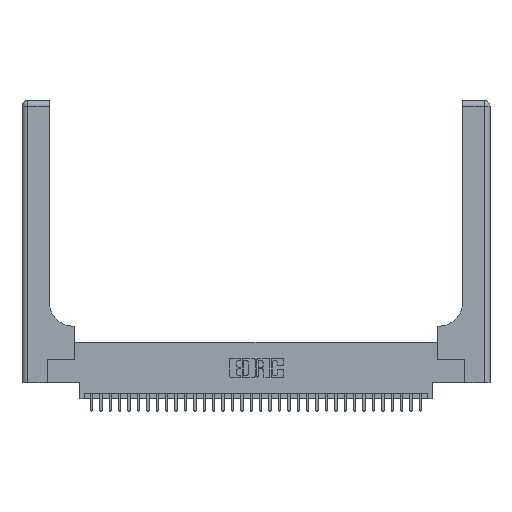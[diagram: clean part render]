
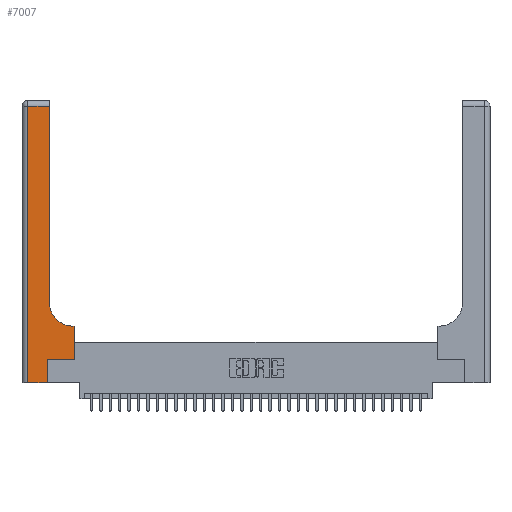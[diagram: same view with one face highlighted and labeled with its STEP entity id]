
A CAD part, top view. The second image highlights one B-rep face of the part: STEP entity #7007.
In plain terms, the highlighted planar face has unit normal (0, 0, 1).
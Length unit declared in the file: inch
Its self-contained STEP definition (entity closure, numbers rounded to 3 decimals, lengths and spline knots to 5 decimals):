
#352 = VERTEX_POINT ( 'NONE', #7722 ) ;
#525 = LINE ( 'NONE', #23520, #14039 ) ;
#1708 = EDGE_CURVE ( 'NONE', #20047, #33948, #4391, .T. ) ;
#1939 = CARTESIAN_POINT ( 'NONE',  ( 0.5415, 0.85, 0.37 ) ) ;
#2057 = ORIENTED_EDGE ( 'NONE', *, *, #12506, .T. ) ;
#2086 = EDGE_CURVE ( 'NONE', #19083, #32326, #525, .T. ) ;
#2488 = CARTESIAN_POINT ( 'NONE',  ( 0.269, 0.25, 0.37 ) ) ;
#2532 = CARTESIAN_POINT ( 'NONE',  ( 0.06, 3., 0.37 ) ) ;
#2657 = CARTESIAN_POINT ( 'NONE',  ( 0., 0., 0.37 ) ) ;
#2663 = DIRECTION ( 'NONE',  ( -1., 0., 0. ) ) ;
#2876 = PLANE ( 'NONE',  #28802 ) ;
#3325 = VERTEX_POINT ( 'NONE', #22741 ) ;
#3393 = VECTOR ( 'NONE', #24776, 39.37008 ) ;
#3789 = CARTESIAN_POINT ( 'NONE',  ( 0.06, 0., 0.37 ) ) ;
#3980 = CARTESIAN_POINT ( 'NONE',  ( 0.5585, 0.25, 0.37 ) ) ;
#4391 = LINE ( 'NONE', #14346, #11543 ) ;
#4538 = VECTOR ( 'NONE', #31846, 39.37008 ) ;
#4563 = VECTOR ( 'NONE', #21100, 39.37008 ) ;
#4647 = DIRECTION ( 'NONE',  ( 1., 0., 0. ) ) ;
#5018 = CARTESIAN_POINT ( 'NONE',  ( 0.269, 0., 0.37 ) ) ;
#5174 = CARTESIAN_POINT ( 'NONE',  ( 0., 2.94, 0.37 ) ) ;
#5252 = DIRECTION ( 'NONE',  ( 0., -1., 0. ) ) ;
#5382 = LINE ( 'NONE', #2657, #4538 ) ;
#5566 = CARTESIAN_POINT ( 'NONE',  ( 0., 3., 0.37 ) ) ;
#6592 = CARTESIAN_POINT ( 'NONE',  ( 0.2915, 2.94, 0.37 ) ) ;
#7007 = ADVANCED_FACE ( 'NONE', ( #11582 ), #2876, .F. ) ;
#7722 = CARTESIAN_POINT ( 'NONE',  ( 0.5585, 0.6, 0.37 ) ) ;
#9692 = LINE ( 'NONE', #3980, #3393 ) ;
#10272 = AXIS2_PLACEMENT_3D ( 'NONE', #1939, #20592, #4647 ) ;
#10968 = DIRECTION ( 'NONE',  ( 0., 0., -1. ) ) ;
#11543 = VECTOR ( 'NONE', #27429, 39.37008 ) ;
#11582 = FACE_OUTER_BOUND ( 'NONE', #27675, .T. ) ;
#11828 = VERTEX_POINT ( 'NONE', #3789 ) ;
#11848 = VECTOR ( 'NONE', #23611, 39.37008 ) ;
#12060 = ORIENTED_EDGE ( 'NONE', *, *, #1708, .T. ) ;
#12506 = EDGE_CURVE ( 'NONE', #32326, #352, #9692, .T. ) ;
#12811 = EDGE_CURVE ( 'NONE', #352, #3325, #21670, .T. ) ;
#13978 = CARTESIAN_POINT ( 'NONE',  ( 0.5585, 0.25, 0.37 ) ) ;
#14039 = VECTOR ( 'NONE', #26137, 39.37008 ) ;
#14093 = EDGE_CURVE ( 'NONE', #11828, #29921, #5382, .T. ) ;
#14346 = CARTESIAN_POINT ( 'NONE',  ( 0.2915, 3., 0.37 ) ) ;
#14990 = VERTEX_POINT ( 'NONE', #17540 ) ;
#15400 = ORIENTED_EDGE ( 'NONE', *, *, #21527, .T. ) ;
#15858 = ORIENTED_EDGE ( 'NONE', *, *, #2086, .T. ) ;
#16429 = ORIENTED_EDGE ( 'NONE', *, *, #25952, .T. ) ;
#16686 = ORIENTED_EDGE ( 'NONE', *, *, #12811, .T. ) ;
#17540 = CARTESIAN_POINT ( 'NONE',  ( 0.06, 2.94, 0.37 ) ) ;
#18045 = LINE ( 'NONE', #5018, #11848 ) ;
#19083 = VERTEX_POINT ( 'NONE', #2488 ) ;
#19380 = ORIENTED_EDGE ( 'NONE', *, *, #14093, .T. ) ;
#19407 = ORIENTED_EDGE ( 'NONE', *, *, #32744, .T. ) ;
#20047 = VERTEX_POINT ( 'NONE', #33692 ) ;
#20592 = DIRECTION ( 'NONE',  ( 0., 0., -1. ) ) ;
#21100 = DIRECTION ( 'NONE',  ( -1., 0., 0. ) ) ;
#21527 = EDGE_CURVE ( 'NONE', #33948, #14990, #25738, .T. ) ;
#21670 = LINE ( 'NONE', #34378, #27040 ) ;
#22741 = CARTESIAN_POINT ( 'NONE',  ( 0.5415, 0.6, 0.37 ) ) ;
#23520 = CARTESIAN_POINT ( 'NONE',  ( 0.269, 0.25, 0.37 ) ) ;
#23611 = DIRECTION ( 'NONE',  ( 0., 1., 0. ) ) ;
#24776 = DIRECTION ( 'NONE',  ( 0., 1., 0. ) ) ;
#25738 = LINE ( 'NONE', #5174, #4563 ) ;
#25952 = EDGE_CURVE ( 'NONE', #3325, #20047, #28066, .T. ) ;
#26137 = DIRECTION ( 'NONE',  ( 1., 0., 0. ) ) ;
#27040 = VECTOR ( 'NONE', #2663, 39.37008 ) ;
#27429 = DIRECTION ( 'NONE',  ( 0., 1., 0. ) ) ;
#27675 = EDGE_LOOP ( 'NONE', ( #12060, #15400, #28806, #19380, #19407, #15858, #2057, #16686, #16429 ) ) ;
#28066 = CIRCLE ( 'NONE', #10272, 0.25 ) ;
#28802 = AXIS2_PLACEMENT_3D ( 'NONE', #5566, #10968, #29420 ) ;
#28806 = ORIENTED_EDGE ( 'NONE', *, *, #32795, .T. ) ;
#29420 = DIRECTION ( 'NONE',  ( -1., 0., 0. ) ) ;
#29921 = VERTEX_POINT ( 'NONE', #30551 ) ;
#30350 = VECTOR ( 'NONE', #5252, 39.37008 ) ;
#30551 = CARTESIAN_POINT ( 'NONE',  ( 0.269, 0., 0.37 ) ) ;
#31181 = LINE ( 'NONE', #2532, #30350 ) ;
#31846 = DIRECTION ( 'NONE',  ( 1., 0., 0. ) ) ;
#32326 = VERTEX_POINT ( 'NONE', #13978 ) ;
#32744 = EDGE_CURVE ( 'NONE', #29921, #19083, #18045, .T. ) ;
#32795 = EDGE_CURVE ( 'NONE', #14990, #11828, #31181, .T. ) ;
#33692 = CARTESIAN_POINT ( 'NONE',  ( 0.2915, 0.85, 0.37 ) ) ;
#33948 = VERTEX_POINT ( 'NONE', #6592 ) ;
#34378 = CARTESIAN_POINT ( 'NONE',  ( 0.2915, 0.6, 0.37 ) ) ;
